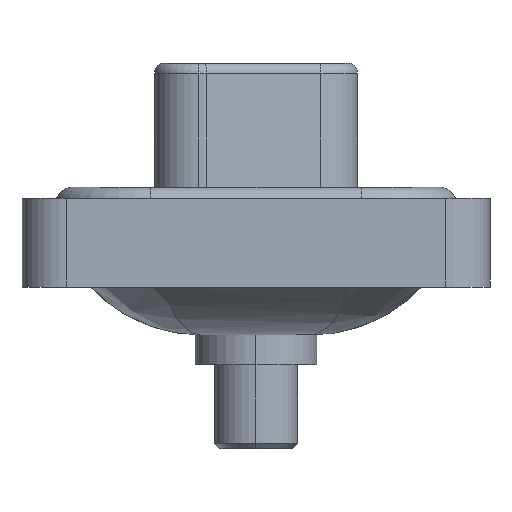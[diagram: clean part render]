
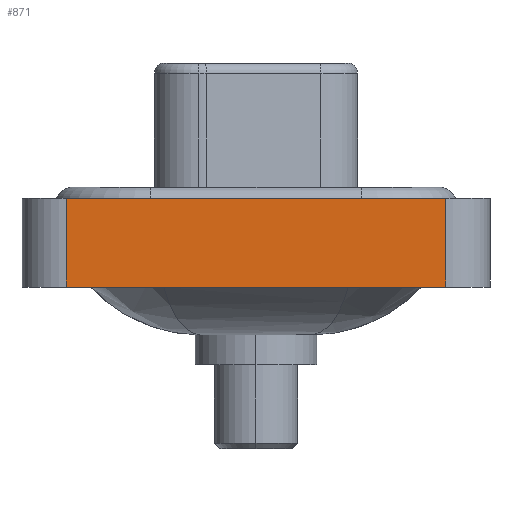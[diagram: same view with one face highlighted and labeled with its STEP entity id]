
A CAD part, left-side view. The second image highlights one B-rep face of the part: STEP entity #871.
In plain terms, the highlighted planar face has unit normal (-1, 0, 0).
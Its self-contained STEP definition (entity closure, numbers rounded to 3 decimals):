
#359 = LINE ( 'NONE', #4446, #11184 ) ;
#367 = CARTESIAN_POINT ( 'NONE',  ( -7.25, 8.55, -3.6 ) ) ;
#871 = ADVANCED_FACE ( 'NONE', ( #15164 ), #2806, .T. ) ;
#1024 = LINE ( 'NONE', #16303, #11295 ) ;
#1808 = EDGE_CURVE ( 'NONE', #10728, #11396, #3106, .T. ) ;
#2223 = VECTOR ( 'NONE', #6122, 1000. ) ;
#2806 = PLANE ( 'NONE',  #12613 ) ;
#3106 = LINE ( 'NONE', #367, #8312 ) ;
#4259 = DIRECTION ( 'NONE',  ( -1., 0., 0. ) ) ;
#4446 = CARTESIAN_POINT ( 'NONE',  ( -7.25, -8.55, 0.4 ) ) ;
#5486 = DIRECTION ( 'NONE',  ( 0., -1., 0. ) ) ;
#5490 = CARTESIAN_POINT ( 'NONE',  ( -7.25, -8.55, -3.6 ) ) ;
#5621 = CARTESIAN_POINT ( 'NONE',  ( -7.25, -8.55, -3.6 ) ) ;
#6122 = DIRECTION ( 'NONE',  ( 0., 0., 1. ) ) ;
#7830 = CARTESIAN_POINT ( 'NONE',  ( -7.25, 8.55, 0.4 ) ) ;
#8002 = EDGE_CURVE ( 'NONE', #9694, #17070, #14206, .T. ) ;
#8148 = EDGE_LOOP ( 'NONE', ( #9211, #8728, #11318, #9478 ) ) ;
#8312 = VECTOR ( 'NONE', #17122, 1000. ) ;
#8728 = ORIENTED_EDGE ( 'NONE', *, *, #15627, .F. ) ;
#8772 = CARTESIAN_POINT ( 'NONE',  ( -7.25, -8.55, 0.4 ) ) ;
#9211 = ORIENTED_EDGE ( 'NONE', *, *, #8002, .T. ) ;
#9478 = ORIENTED_EDGE ( 'NONE', *, *, #13701, .T. ) ;
#9694 = VERTEX_POINT ( 'NONE', #5490 ) ;
#10185 = DIRECTION ( 'NONE',  ( 0., -1., 0. ) ) ;
#10728 = VERTEX_POINT ( 'NONE', #16179 ) ;
#10991 = DIRECTION ( 'NONE',  ( 0., 0., 1. ) ) ;
#11184 = VECTOR ( 'NONE', #10185, 1000. ) ;
#11295 = VECTOR ( 'NONE', #5486, 1000. ) ;
#11318 = ORIENTED_EDGE ( 'NONE', *, *, #1808, .F. ) ;
#11396 = VERTEX_POINT ( 'NONE', #7830 ) ;
#12613 = AXIS2_PLACEMENT_3D ( 'NONE', #5621, #4259, #10991 ) ;
#13026 = CARTESIAN_POINT ( 'NONE',  ( -7.25, -8.55, -3.6 ) ) ;
#13701 = EDGE_CURVE ( 'NONE', #10728, #9694, #1024, .T. ) ;
#14206 = LINE ( 'NONE', #13026, #2223 ) ;
#15164 = FACE_OUTER_BOUND ( 'NONE', #8148, .T. ) ;
#15627 = EDGE_CURVE ( 'NONE', #11396, #17070, #359, .T. ) ;
#16179 = CARTESIAN_POINT ( 'NONE',  ( -7.25, 8.55, -3.6 ) ) ;
#16303 = CARTESIAN_POINT ( 'NONE',  ( -7.25, -8.55, -3.6 ) ) ;
#17070 = VERTEX_POINT ( 'NONE', #8772 ) ;
#17122 = DIRECTION ( 'NONE',  ( 0., 0., 1. ) ) ;
